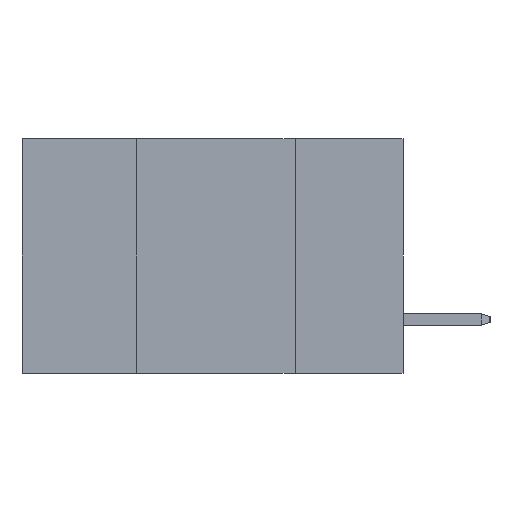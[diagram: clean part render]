
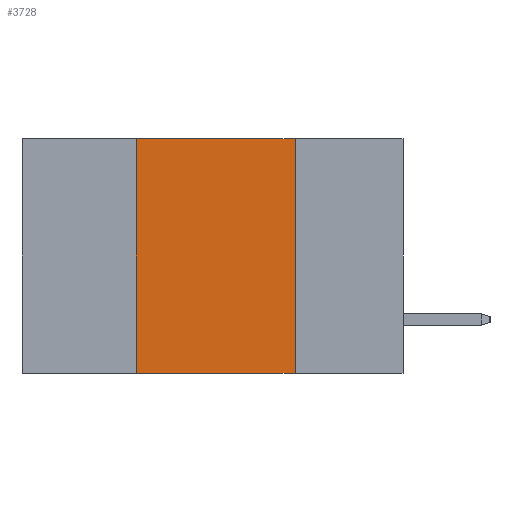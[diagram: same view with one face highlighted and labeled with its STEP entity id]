
A CAD part, left-side view. The second image highlights one B-rep face of the part: STEP entity #3728.
In plain terms, the highlighted planar face has unit normal (-1, 0, 0).
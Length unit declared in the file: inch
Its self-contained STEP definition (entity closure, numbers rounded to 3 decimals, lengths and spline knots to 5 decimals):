
#716 = LINE ( 'NONE', #3407, #10216 ) ;
#1177 = VERTEX_POINT ( 'NONE', #11182 ) ;
#1259 = LINE ( 'NONE', #2985, #8049 ) ;
#1552 = VECTOR ( 'NONE', #7001, 39.37008 ) ;
#1716 = EDGE_CURVE ( 'NONE', #1177, #9996, #3826, .T. ) ;
#2116 = PLANE ( 'NONE',  #6315 ) ;
#2322 = VERTEX_POINT ( 'NONE', #6566 ) ;
#2336 = ORIENTED_EDGE ( 'NONE', *, *, #6888, .F. ) ;
#2479 = ORIENTED_EDGE ( 'NONE', *, *, #7207, .F. ) ;
#2689 = ORIENTED_EDGE ( 'NONE', *, *, #1716, .T. ) ;
#2969 = DIRECTION ( 'NONE',  ( 0., 0., -1. ) ) ;
#2985 = CARTESIAN_POINT ( 'NONE',  ( 0., 0.17, 0. ) ) ;
#3188 = VERTEX_POINT ( 'NONE', #3488 ) ;
#3407 = CARTESIAN_POINT ( 'NONE',  ( 0., 0.42, 0. ) ) ;
#3488 = CARTESIAN_POINT ( 'NONE',  ( 0., 0.17, 0. ) ) ;
#3715 = ORIENTED_EDGE ( 'NONE', *, *, #8244, .F. ) ;
#3728 = ADVANCED_FACE ( 'NONE', ( #7584 ), #2116, .F. ) ;
#3826 = LINE ( 'NONE', #5450, #7580 ) ;
#5450 = CARTESIAN_POINT ( 'NONE',  ( 0., 0.6, -0.37 ) ) ;
#5677 = CARTESIAN_POINT ( 'NONE',  ( 0., 0.6, 0. ) ) ;
#6315 = AXIS2_PLACEMENT_3D ( 'NONE', #5677, #9191, #2969 ) ;
#6566 = CARTESIAN_POINT ( 'NONE',  ( 0., 0.42, 0. ) ) ;
#6888 = EDGE_CURVE ( 'NONE', #1177, #2322, #716, .T. ) ;
#7001 = DIRECTION ( 'NONE',  ( 0., -1., 0. ) ) ;
#7159 = EDGE_LOOP ( 'NONE', ( #2479, #3715, #2336, #2689 ) ) ;
#7207 = EDGE_CURVE ( 'NONE', #3188, #9996, #1259, .T. ) ;
#7580 = VECTOR ( 'NONE', #10850, 39.37008 ) ;
#7584 = FACE_OUTER_BOUND ( 'NONE', #7159, .T. ) ;
#7882 = CARTESIAN_POINT ( 'NONE',  ( 0., 0.6, 0. ) ) ;
#7987 = CARTESIAN_POINT ( 'NONE',  ( 0., 0.17, -0.37 ) ) ;
#8024 = DIRECTION ( 'NONE',  ( 0., 0., 1. ) ) ;
#8049 = VECTOR ( 'NONE', #10000, 39.37008 ) ;
#8244 = EDGE_CURVE ( 'NONE', #2322, #3188, #9591, .T. ) ;
#9191 = DIRECTION ( 'NONE',  ( 1., 0., 0. ) ) ;
#9591 = LINE ( 'NONE', #7882, #1552 ) ;
#9996 = VERTEX_POINT ( 'NONE', #7987 ) ;
#10000 = DIRECTION ( 'NONE',  ( 0., 0., -1. ) ) ;
#10216 = VECTOR ( 'NONE', #8024, 39.37008 ) ;
#10850 = DIRECTION ( 'NONE',  ( 0., -1., 0. ) ) ;
#11182 = CARTESIAN_POINT ( 'NONE',  ( 0., 0.42, -0.37 ) ) ;
